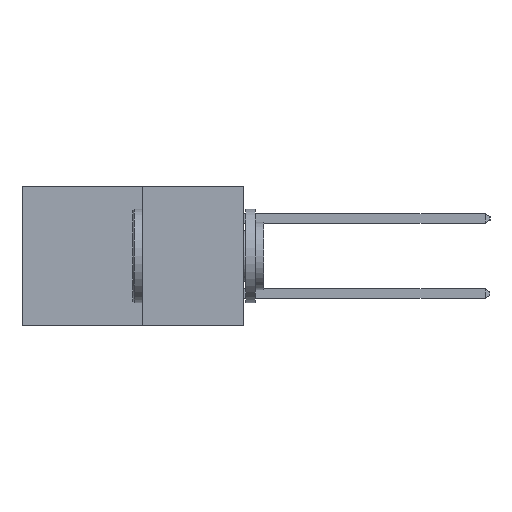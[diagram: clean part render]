
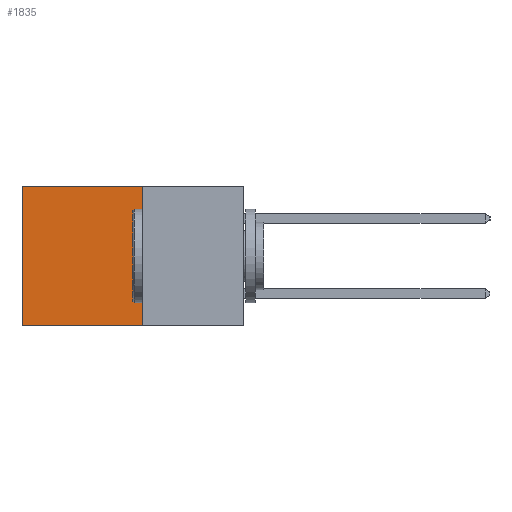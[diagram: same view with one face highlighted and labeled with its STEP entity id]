
A CAD part, left-side view. The second image highlights one B-rep face of the part: STEP entity #1835.
In plain terms, the highlighted planar face has unit normal (-1, 0, 0).
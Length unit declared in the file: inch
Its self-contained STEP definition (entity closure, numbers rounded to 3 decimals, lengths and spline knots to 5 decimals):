
#324 = LINE ( 'NONE', #6201, #2334 ) ;
#812 = EDGE_CURVE ( 'NONE', #5450, #2119, #6150, .T. ) ;
#1326 = EDGE_CURVE ( 'NONE', #5860, #4713, #6957, .T. ) ;
#1356 = CARTESIAN_POINT ( 'NONE',  ( 0.277, 0.27, -0.37 ) ) ;
#1835 = ADVANCED_FACE ( 'NONE', ( #3953 ), #7795, .F. ) ;
#2119 = VERTEX_POINT ( 'NONE', #8538 ) ;
#2334 = VECTOR ( 'NONE', #6231, 39.37008 ) ;
#2823 = VECTOR ( 'NONE', #6226, 39.37008 ) ;
#3043 = LINE ( 'NONE', #6307, #2823 ) ;
#3334 = CARTESIAN_POINT ( 'NONE',  ( 0.277, 0.27, -0.37 ) ) ;
#3582 = ORIENTED_EDGE ( 'NONE', *, *, #1326, .T. ) ;
#3918 = EDGE_CURVE ( 'NONE', #5860, #5450, #3043, .T. ) ;
#3953 = FACE_OUTER_BOUND ( 'NONE', #8596, .T. ) ;
#4678 = CARTESIAN_POINT ( 'NONE',  ( 0.277, 0.59, 0. ) ) ;
#4713 = VERTEX_POINT ( 'NONE', #4678 ) ;
#4967 = CARTESIAN_POINT ( 'NONE',  ( 0.277, 0.27, -0.37 ) ) ;
#5167 = VECTOR ( 'NONE', #5280, 39.37008 ) ;
#5280 = DIRECTION ( 'NONE',  ( 0., 1., 0. ) ) ;
#5450 = VERTEX_POINT ( 'NONE', #3334 ) ;
#5597 = CARTESIAN_POINT ( 'NONE',  ( 0.277, 0.27, 0. ) ) ;
#5613 = AXIS2_PLACEMENT_3D ( 'NONE', #4967, #8189, #6659 ) ;
#5860 = VERTEX_POINT ( 'NONE', #7437 ) ;
#5935 = VECTOR ( 'NONE', #7430, 39.37008 ) ;
#6061 = EDGE_CURVE ( 'NONE', #4713, #2119, #324, .T. ) ;
#6150 = LINE ( 'NONE', #1356, #5935 ) ;
#6201 = CARTESIAN_POINT ( 'NONE',  ( 0.277, 0.59, -0.37 ) ) ;
#6226 = DIRECTION ( 'NONE',  ( 0., 0., -1. ) ) ;
#6231 = DIRECTION ( 'NONE',  ( 0., 0., -1. ) ) ;
#6307 = CARTESIAN_POINT ( 'NONE',  ( 0.277, 0.27, -0.37 ) ) ;
#6513 = ORIENTED_EDGE ( 'NONE', *, *, #6061, .T. ) ;
#6659 = DIRECTION ( 'NONE',  ( 0., 0., -1. ) ) ;
#6919 = ORIENTED_EDGE ( 'NONE', *, *, #3918, .F. ) ;
#6957 = LINE ( 'NONE', #5597, #5167 ) ;
#7430 = DIRECTION ( 'NONE',  ( 0., 1., 0. ) ) ;
#7437 = CARTESIAN_POINT ( 'NONE',  ( 0.277, 0.27, 0. ) ) ;
#7795 = PLANE ( 'NONE',  #5613 ) ;
#8189 = DIRECTION ( 'NONE',  ( 1., 0., 0. ) ) ;
#8460 = ORIENTED_EDGE ( 'NONE', *, *, #812, .F. ) ;
#8538 = CARTESIAN_POINT ( 'NONE',  ( 0.277, 0.59, -0.37 ) ) ;
#8596 = EDGE_LOOP ( 'NONE', ( #6513, #8460, #6919, #3582 ) ) ;
